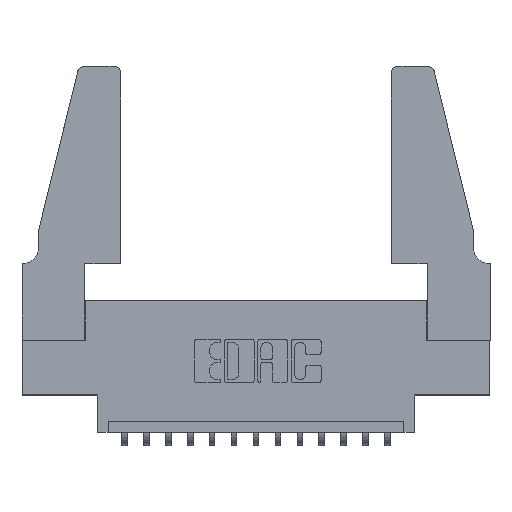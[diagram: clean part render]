
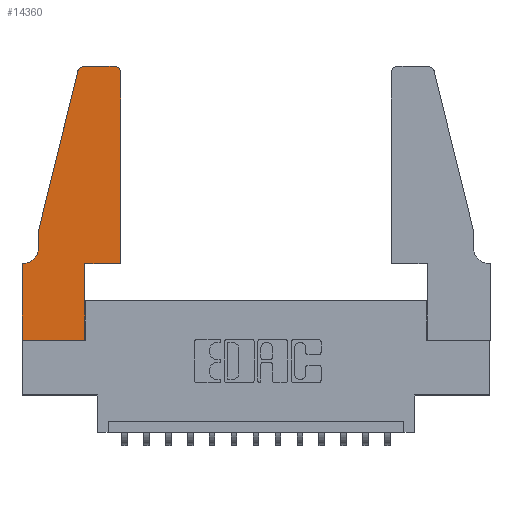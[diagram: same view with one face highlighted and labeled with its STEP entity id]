
A CAD part, top view. The second image highlights one B-rep face of the part: STEP entity #14360.
In plain terms, the highlighted planar face has unit normal (0, 0, 1).
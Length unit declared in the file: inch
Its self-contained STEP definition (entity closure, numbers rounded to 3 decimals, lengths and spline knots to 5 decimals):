
#112 = DIRECTION ( 'NONE',  ( 1., 0., 0. ) ) ;
#119 = ORIENTED_EDGE ( 'NONE', *, *, #12644, .T. ) ;
#134 = VERTEX_POINT ( 'NONE', #11441 ) ;
#162 = CARTESIAN_POINT ( 'NONE',  ( 0., 0., 0.37 ) ) ;
#650 = VECTOR ( 'NONE', #2553, 39.37008 ) ;
#1309 = CARTESIAN_POINT ( 'NONE',  ( 0.2865, 0.35, 0.37 ) ) ;
#1484 = CARTESIAN_POINT ( 'NONE',  ( 0.2605, 1.25, 0.37 ) ) ;
#2030 = VERTEX_POINT ( 'NONE', #4282 ) ;
#2080 = DIRECTION ( 'NONE',  ( 0., 1., 0. ) ) ;
#2113 = LINE ( 'NONE', #2243, #11846 ) ;
#2196 = ORIENTED_EDGE ( 'NONE', *, *, #15214, .T. ) ;
#2243 = CARTESIAN_POINT ( 'NONE',  ( 0.4505, 0.35, 0.37 ) ) ;
#2434 = CARTESIAN_POINT ( 'NONE',  ( 0.0055, 0.42, 0.37 ) ) ;
#2553 = DIRECTION ( 'NONE',  ( 0., -1., 0. ) ) ;
#2572 = ORIENTED_EDGE ( 'NONE', *, *, #11313, .T. ) ;
#2734 = DIRECTION ( 'NONE',  ( -1., 0., 0. ) ) ;
#2754 = ORIENTED_EDGE ( 'NONE', *, *, #6927, .T. ) ;
#3030 = EDGE_CURVE ( 'NONE', #3337, #8929, #10049, .T. ) ;
#3221 = FACE_OUTER_BOUND ( 'NONE', #14156, .T. ) ;
#3337 = VERTEX_POINT ( 'NONE', #10959 ) ;
#3379 = LINE ( 'NONE', #10314, #6726 ) ;
#3404 = CARTESIAN_POINT ( 'NONE',  ( 0.4205, 1.22, 0.37 ) ) ;
#3559 = EDGE_CURVE ( 'NONE', #2030, #14997, #10215, .T. ) ;
#3587 = LINE ( 'NONE', #5011, #650 ) ;
#3675 = DIRECTION ( 'NONE',  ( 0., 1., 0. ) ) ;
#3709 = CARTESIAN_POINT ( 'NONE',  ( 0., 0.35, 0.37 ) ) ;
#3820 = CARTESIAN_POINT ( 'NONE',  ( 0., 0.35, 0.37 ) ) ;
#3948 = EDGE_CURVE ( 'NONE', #8929, #15947, #5723, .T. ) ;
#4282 = CARTESIAN_POINT ( 'NONE',  ( 0.2865, 0.35, 0.37 ) ) ;
#4672 = VERTEX_POINT ( 'NONE', #7882 ) ;
#4952 = CARTESIAN_POINT ( 'NONE',  ( 0.284, 1.22, 0.37 ) ) ;
#5011 = CARTESIAN_POINT ( 'NONE',  ( 0., 0., 0.37 ) ) ;
#5101 = CARTESIAN_POINT ( 'NONE',  ( 0.2865, 0., 0.37 ) ) ;
#5108 = DIRECTION ( 'NONE',  ( 1., 0., 0. ) ) ;
#5230 = DIRECTION ( 'NONE',  ( 0., 0., 1. ) ) ;
#5621 = AXIS2_PLACEMENT_3D ( 'NONE', #2434, #13668, #7638 ) ;
#5723 = LINE ( 'NONE', #7895, #12116 ) ;
#5823 = CARTESIAN_POINT ( 'NONE',  ( 0.25487, 1.22718, 0.37 ) ) ;
#5914 = LINE ( 'NONE', #7524, #12296 ) ;
#5934 = EDGE_CURVE ( 'NONE', #14997, #4672, #2113, .T. ) ;
#6726 = VECTOR ( 'NONE', #9196, 39.37008 ) ;
#6859 = VECTOR ( 'NONE', #6915, 39.37008 ) ;
#6915 = DIRECTION ( 'NONE',  ( -0.239, -0.971, 0. ) ) ;
#6927 = EDGE_CURVE ( 'NONE', #13386, #134, #11322, .T. ) ;
#7089 = VERTEX_POINT ( 'NONE', #8247 ) ;
#7235 = ORIENTED_EDGE ( 'NONE', *, *, #3948, .T. ) ;
#7303 = AXIS2_PLACEMENT_3D ( 'NONE', #3820, #5230, #15089 ) ;
#7524 = CARTESIAN_POINT ( 'NONE',  ( 0., 0., 0.37 ) ) ;
#7638 = DIRECTION ( 'NONE',  ( -1., 0., 0. ) ) ;
#7714 = PLANE ( 'NONE',  #7303 ) ;
#7754 = ORIENTED_EDGE ( 'NONE', *, *, #8401, .T. ) ;
#7882 = CARTESIAN_POINT ( 'NONE',  ( 0.4505, 1.22, 0.37 ) ) ;
#7895 = CARTESIAN_POINT ( 'NONE',  ( 0.0755, 0.35, 0.37 ) ) ;
#8094 = VECTOR ( 'NONE', #112, 39.37008 ) ;
#8247 = CARTESIAN_POINT ( 'NONE',  ( 0.0755, 0.5, 0.37 ) ) ;
#8296 = EDGE_CURVE ( 'NONE', #10172, #7089, #10542, .T. ) ;
#8401 = EDGE_CURVE ( 'NONE', #7089, #3337, #3379, .T. ) ;
#8633 = ORIENTED_EDGE ( 'NONE', *, *, #3030, .T. ) ;
#8691 = CIRCLE ( 'NONE', #12323, 0.03 ) ;
#8737 = DIRECTION ( 'NONE',  ( 0., 0., 1. ) ) ;
#8929 = VERTEX_POINT ( 'NONE', #10709 ) ;
#8951 = VECTOR ( 'NONE', #3675, 39.37008 ) ;
#9196 = DIRECTION ( 'NONE',  ( 0., -1., 0. ) ) ;
#9573 = CARTESIAN_POINT ( 'NONE',  ( 0.4205, 1.25, 0.37 ) ) ;
#9839 = DIRECTION ( 'NONE',  ( 1., 0., 0. ) ) ;
#9846 = ORIENTED_EDGE ( 'NONE', *, *, #11984, .T. ) ;
#9942 = DIRECTION ( 'NONE',  ( 1., 0., 0. ) ) ;
#10049 = CIRCLE ( 'NONE', #5621, 0.07 ) ;
#10172 = VERTEX_POINT ( 'NONE', #5823 ) ;
#10184 = ORIENTED_EDGE ( 'NONE', *, *, #3559, .T. ) ;
#10215 = LINE ( 'NONE', #14899, #8094 ) ;
#10314 = CARTESIAN_POINT ( 'NONE',  ( 0.0755, 0.5, 0.37 ) ) ;
#10369 = ORIENTED_EDGE ( 'NONE', *, *, #8296, .T. ) ;
#10382 = ORIENTED_EDGE ( 'NONE', *, *, #5934, .T. ) ;
#10502 = LINE ( 'NONE', #1309, #8951 ) ;
#10535 = VERTEX_POINT ( 'NONE', #5101 ) ;
#10542 = LINE ( 'NONE', #14295, #6859 ) ;
#10603 = VERTEX_POINT ( 'NONE', #162 ) ;
#10709 = CARTESIAN_POINT ( 'NONE',  ( 0.0055, 0.35, 0.37 ) ) ;
#10740 = VECTOR ( 'NONE', #2734, 39.37008 ) ;
#10959 = CARTESIAN_POINT ( 'NONE',  ( 0.0755, 0.42, 0.37 ) ) ;
#11004 = DIRECTION ( 'NONE',  ( 0., 0., 1. ) ) ;
#11313 = EDGE_CURVE ( 'NONE', #134, #10172, #8691, .T. ) ;
#11322 = LINE ( 'NONE', #1484, #10740 ) ;
#11345 = CIRCLE ( 'NONE', #15251, 0.03 ) ;
#11441 = CARTESIAN_POINT ( 'NONE',  ( 0.284, 1.25, 0.37 ) ) ;
#11710 = DIRECTION ( 'NONE',  ( -1., 0., 0. ) ) ;
#11846 = VECTOR ( 'NONE', #2080, 39.37008 ) ;
#11984 = EDGE_CURVE ( 'NONE', #10603, #10535, #5914, .T. ) ;
#12116 = VECTOR ( 'NONE', #11710, 39.37008 ) ;
#12296 = VECTOR ( 'NONE', #9942, 39.37008 ) ;
#12323 = AXIS2_PLACEMENT_3D ( 'NONE', #4952, #8737, #5108 ) ;
#12425 = EDGE_CURVE ( 'NONE', #4672, #13386, #11345, .T. ) ;
#12644 = EDGE_CURVE ( 'NONE', #10535, #2030, #10502, .T. ) ;
#13386 = VERTEX_POINT ( 'NONE', #9573 ) ;
#13668 = DIRECTION ( 'NONE',  ( 0., 0., -1. ) ) ;
#13860 = ORIENTED_EDGE ( 'NONE', *, *, #12425, .T. ) ;
#14156 = EDGE_LOOP ( 'NONE', ( #2754, #2572, #10369, #7754, #8633, #7235, #2196, #9846, #119, #10184, #10382, #13860 ) ) ;
#14295 = CARTESIAN_POINT ( 'NONE',  ( 0.0755, 0.5, 0.37 ) ) ;
#14360 = ADVANCED_FACE ( 'NONE', ( #3221 ), #7714, .T. ) ;
#14899 = CARTESIAN_POINT ( 'NONE',  ( 0.4505, 0.35, 0.37 ) ) ;
#14997 = VERTEX_POINT ( 'NONE', #15733 ) ;
#15089 = DIRECTION ( 'NONE',  ( 1., 0., 0. ) ) ;
#15214 = EDGE_CURVE ( 'NONE', #15947, #10603, #3587, .T. ) ;
#15251 = AXIS2_PLACEMENT_3D ( 'NONE', #3404, #11004, #9839 ) ;
#15733 = CARTESIAN_POINT ( 'NONE',  ( 0.4505, 0.35, 0.37 ) ) ;
#15947 = VERTEX_POINT ( 'NONE', #3709 ) ;
